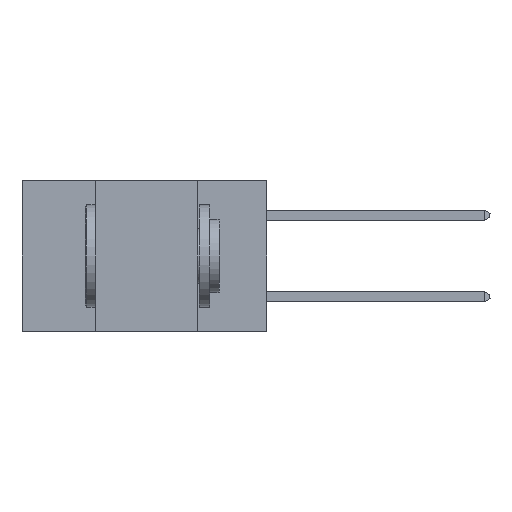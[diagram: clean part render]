
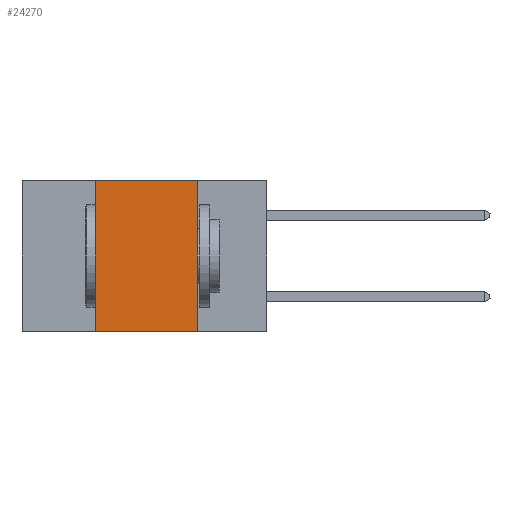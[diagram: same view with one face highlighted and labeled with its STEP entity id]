
A CAD part, left-side view. The second image highlights one B-rep face of the part: STEP entity #24270.
In plain terms, the highlighted planar face has unit normal (-1, 0, 0).
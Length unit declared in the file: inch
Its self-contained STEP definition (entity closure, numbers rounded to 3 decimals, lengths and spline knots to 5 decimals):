
#178 = EDGE_CURVE ( 'NONE', #33379, #21437, #21007, .T. ) ;
#1875 = CARTESIAN_POINT ( 'NONE',  ( 0., 0.17, 0. ) ) ;
#2407 = FACE_OUTER_BOUND ( 'NONE', #17273, .T. ) ;
#3922 = EDGE_CURVE ( 'NONE', #15883, #18241, #28790, .T. ) ;
#5175 = ORIENTED_EDGE ( 'NONE', *, *, #21433, .T. ) ;
#5836 = VECTOR ( 'NONE', #18419, 39.37008 ) ;
#6311 = VECTOR ( 'NONE', #13716, 39.37008 ) ;
#7103 = CARTESIAN_POINT ( 'NONE',  ( 0., 0.6, -0.37 ) ) ;
#10567 = CARTESIAN_POINT ( 'NONE',  ( 0., 0.6, 0. ) ) ;
#11866 = CARTESIAN_POINT ( 'NONE',  ( 0., 0.6, 0. ) ) ;
#12360 = DIRECTION ( 'NONE',  ( 0., -1., 0. ) ) ;
#13716 = DIRECTION ( 'NONE',  ( 0., 0., -1. ) ) ;
#14083 = EDGE_CURVE ( 'NONE', #18241, #33379, #19726, .T. ) ;
#14506 = DIRECTION ( 'NONE',  ( 0., 0., -1. ) ) ;
#14529 = DIRECTION ( 'NONE',  ( 0., 0., 1. ) ) ;
#15752 = VECTOR ( 'NONE', #14529, 39.37008 ) ;
#15883 = VERTEX_POINT ( 'NONE', #25872 ) ;
#17273 = EDGE_LOOP ( 'NONE', ( #24764, #18618, #32033, #5175 ) ) ;
#18241 = VERTEX_POINT ( 'NONE', #21706 ) ;
#18267 = CARTESIAN_POINT ( 'NONE',  ( 0., 0.17, 0. ) ) ;
#18419 = DIRECTION ( 'NONE',  ( 0., -1., 0. ) ) ;
#18618 = ORIENTED_EDGE ( 'NONE', *, *, #14083, .F. ) ;
#19726 = LINE ( 'NONE', #10567, #5836 ) ;
#21007 = LINE ( 'NONE', #18267, #6311 ) ;
#21433 = EDGE_CURVE ( 'NONE', #15883, #21437, #29884, .T. ) ;
#21437 = VERTEX_POINT ( 'NONE', #27977 ) ;
#21706 = CARTESIAN_POINT ( 'NONE',  ( 0., 0.42, 0. ) ) ;
#22136 = VECTOR ( 'NONE', #12360, 39.37008 ) ;
#24177 = AXIS2_PLACEMENT_3D ( 'NONE', #11866, #30078, #14506 ) ;
#24270 = ADVANCED_FACE ( 'NONE', ( #2407 ), #24871, .F. ) ;
#24764 = ORIENTED_EDGE ( 'NONE', *, *, #178, .F. ) ;
#24871 = PLANE ( 'NONE',  #24177 ) ;
#25872 = CARTESIAN_POINT ( 'NONE',  ( 0., 0.42, -0.37 ) ) ;
#27977 = CARTESIAN_POINT ( 'NONE',  ( 0., 0.17, -0.37 ) ) ;
#28790 = LINE ( 'NONE', #30096, #15752 ) ;
#29884 = LINE ( 'NONE', #7103, #22136 ) ;
#30078 = DIRECTION ( 'NONE',  ( 1., 0., 0. ) ) ;
#30096 = CARTESIAN_POINT ( 'NONE',  ( 0., 0.42, 0. ) ) ;
#32033 = ORIENTED_EDGE ( 'NONE', *, *, #3922, .F. ) ;
#33379 = VERTEX_POINT ( 'NONE', #1875 ) ;
